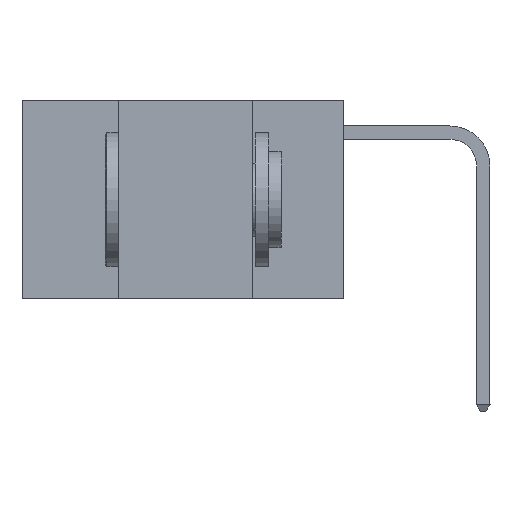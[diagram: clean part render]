
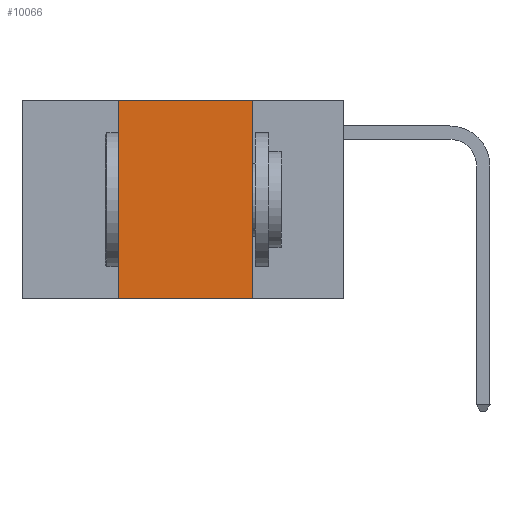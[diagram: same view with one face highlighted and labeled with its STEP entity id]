
A CAD part, left-side view. The second image highlights one B-rep face of the part: STEP entity #10066.
In plain terms, the highlighted planar face has unit normal (-1, 0, 0).
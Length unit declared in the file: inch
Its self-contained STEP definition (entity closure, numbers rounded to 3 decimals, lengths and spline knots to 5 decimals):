
#361 = ORIENTED_EDGE ( 'NONE', *, *, #9721, .F. ) ;
#671 = DIRECTION ( 'NONE',  ( 1., 0., 0. ) ) ;
#877 = LINE ( 'NONE', #4088, #6424 ) ;
#941 = CARTESIAN_POINT ( 'NONE',  ( 0., 0.17, 0. ) ) ;
#1191 = VECTOR ( 'NONE', #2016, 39.37008 ) ;
#1669 = VECTOR ( 'NONE', #3178, 39.37008 ) ;
#1808 = CARTESIAN_POINT ( 'NONE',  ( 0., 0.6, 0. ) ) ;
#1814 = CARTESIAN_POINT ( 'NONE',  ( 0., 0.17, 0. ) ) ;
#2016 = DIRECTION ( 'NONE',  ( 0., -1., 0. ) ) ;
#2453 = ORIENTED_EDGE ( 'NONE', *, *, #11145, .F. ) ;
#3178 = DIRECTION ( 'NONE',  ( 0., 0., 1. ) ) ;
#3399 = LINE ( 'NONE', #941, #3791 ) ;
#3791 = VECTOR ( 'NONE', #5565, 39.37008 ) ;
#4088 = CARTESIAN_POINT ( 'NONE',  ( 0., 0.6, 0. ) ) ;
#4274 = LINE ( 'NONE', #13401, #1669 ) ;
#5031 = ORIENTED_EDGE ( 'NONE', *, *, #9684, .F. ) ;
#5223 = VERTEX_POINT ( 'NONE', #6171 ) ;
#5565 = DIRECTION ( 'NONE',  ( 0., 0., -1. ) ) ;
#6171 = CARTESIAN_POINT ( 'NONE',  ( 0., 0.42, -0.37 ) ) ;
#6424 = VECTOR ( 'NONE', #8741, 39.37008 ) ;
#6844 = CARTESIAN_POINT ( 'NONE',  ( 0., 0.6, -0.37 ) ) ;
#7161 = PLANE ( 'NONE',  #12108 ) ;
#7696 = VERTEX_POINT ( 'NONE', #8859 ) ;
#8095 = EDGE_LOOP ( 'NONE', ( #361, #2453, #5031, #14551 ) ) ;
#8741 = DIRECTION ( 'NONE',  ( 0., -1., 0. ) ) ;
#8859 = CARTESIAN_POINT ( 'NONE',  ( 0., 0.17, -0.37 ) ) ;
#9620 = VERTEX_POINT ( 'NONE', #10355 ) ;
#9684 = EDGE_CURVE ( 'NONE', #5223, #9620, #4274, .T. ) ;
#9721 = EDGE_CURVE ( 'NONE', #14327, #7696, #3399, .T. ) ;
#10066 = ADVANCED_FACE ( 'NONE', ( #14224 ), #7161, .F. ) ;
#10355 = CARTESIAN_POINT ( 'NONE',  ( 0., 0.42, 0. ) ) ;
#10791 = EDGE_CURVE ( 'NONE', #5223, #7696, #11323, .T. ) ;
#11145 = EDGE_CURVE ( 'NONE', #9620, #14327, #877, .T. ) ;
#11323 = LINE ( 'NONE', #6844, #1191 ) ;
#11988 = DIRECTION ( 'NONE',  ( 0., 0., -1. ) ) ;
#12108 = AXIS2_PLACEMENT_3D ( 'NONE', #1808, #671, #11988 ) ;
#13401 = CARTESIAN_POINT ( 'NONE',  ( 0., 0.42, 0. ) ) ;
#14224 = FACE_OUTER_BOUND ( 'NONE', #8095, .T. ) ;
#14327 = VERTEX_POINT ( 'NONE', #1814 ) ;
#14551 = ORIENTED_EDGE ( 'NONE', *, *, #10791, .T. ) ;
